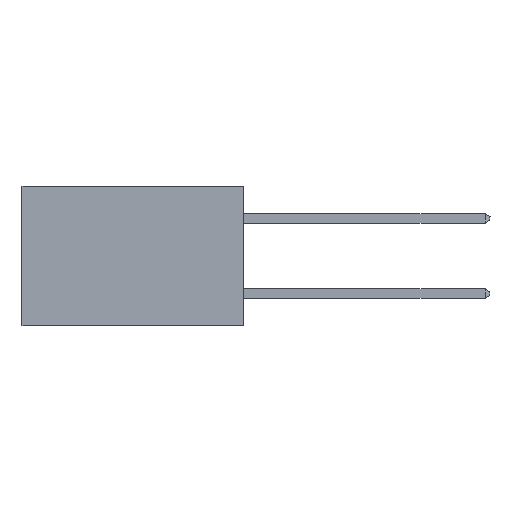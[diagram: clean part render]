
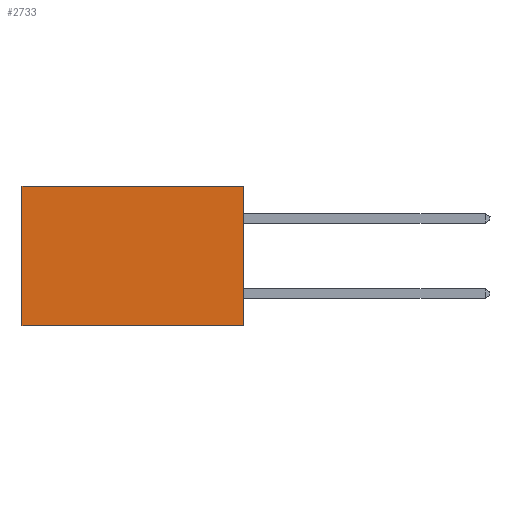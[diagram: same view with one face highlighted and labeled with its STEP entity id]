
A CAD part, left-side view. The second image highlights one B-rep face of the part: STEP entity #2733.
In plain terms, the highlighted planar face has unit normal (-1, 0, 0).
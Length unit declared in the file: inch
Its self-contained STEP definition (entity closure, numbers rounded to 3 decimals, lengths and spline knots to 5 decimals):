
#336 = ORIENTED_EDGE ( 'NONE', *, *, #2800, .F. ) ;
#1606 = CARTESIAN_POINT ( 'NONE',  ( 0.277, 0., -0.37 ) ) ;
#1655 = ORIENTED_EDGE ( 'NONE', *, *, #14905, .T. ) ;
#1852 = EDGE_CURVE ( 'NONE', #22358, #17738, #22630, .T. ) ;
#2131 = LINE ( 'NONE', #22096, #17991 ) ;
#2733 = ADVANCED_FACE ( 'NONE', ( #14017 ), #7130, .F. ) ;
#2800 = EDGE_CURVE ( 'NONE', #5440, #22358, #2131, .T. ) ;
#4137 = CARTESIAN_POINT ( 'NONE',  ( 0.277, 0.59, -0.37 ) ) ;
#5440 = VERTEX_POINT ( 'NONE', #21712 ) ;
#5980 = ORIENTED_EDGE ( 'NONE', *, *, #1852, .F. ) ;
#7130 = PLANE ( 'NONE',  #19633 ) ;
#7374 = DIRECTION ( 'NONE',  ( 0., 0., -1. ) ) ;
#7714 = DIRECTION ( 'NONE',  ( 0., 1., 0. ) ) ;
#7931 = VECTOR ( 'NONE', #7714, 39.37008 ) ;
#8146 = VERTEX_POINT ( 'NONE', #24450 ) ;
#10594 = EDGE_CURVE ( 'NONE', #8146, #17738, #22105, .T. ) ;
#10725 = CARTESIAN_POINT ( 'NONE',  ( 0.277, 0.59, -0.37 ) ) ;
#12167 = DIRECTION ( 'NONE',  ( 0., 0., -1. ) ) ;
#12640 = LINE ( 'NONE', #19552, #7931 ) ;
#14017 = FACE_OUTER_BOUND ( 'NONE', #20706, .T. ) ;
#14021 = DIRECTION ( 'NONE',  ( 0., 0., -1. ) ) ;
#14726 = DIRECTION ( 'NONE',  ( 1., 0., 0. ) ) ;
#14905 = EDGE_CURVE ( 'NONE', #5440, #8146, #12640, .T. ) ;
#15756 = CARTESIAN_POINT ( 'NONE',  ( 0.277, 0., -0.37 ) ) ;
#16905 = VECTOR ( 'NONE', #12167, 39.37008 ) ;
#17738 = VERTEX_POINT ( 'NONE', #10725 ) ;
#17991 = VECTOR ( 'NONE', #7374, 39.37008 ) ;
#18043 = VECTOR ( 'NONE', #19335, 39.37008 ) ;
#18669 = CARTESIAN_POINT ( 'NONE',  ( 0.277, 0., -0.37 ) ) ;
#19335 = DIRECTION ( 'NONE',  ( 0., 1., 0. ) ) ;
#19552 = CARTESIAN_POINT ( 'NONE',  ( 0.277, 0., 0. ) ) ;
#19633 = AXIS2_PLACEMENT_3D ( 'NONE', #15756, #14726, #14021 ) ;
#20706 = EDGE_LOOP ( 'NONE', ( #22596, #5980, #336, #1655 ) ) ;
#21712 = CARTESIAN_POINT ( 'NONE',  ( 0.277, 0., 0. ) ) ;
#22096 = CARTESIAN_POINT ( 'NONE',  ( 0.277, 0., -0.37 ) ) ;
#22105 = LINE ( 'NONE', #4137, #16905 ) ;
#22358 = VERTEX_POINT ( 'NONE', #18669 ) ;
#22596 = ORIENTED_EDGE ( 'NONE', *, *, #10594, .T. ) ;
#22630 = LINE ( 'NONE', #1606, #18043 ) ;
#24450 = CARTESIAN_POINT ( 'NONE',  ( 0.277, 0.59, 0. ) ) ;
